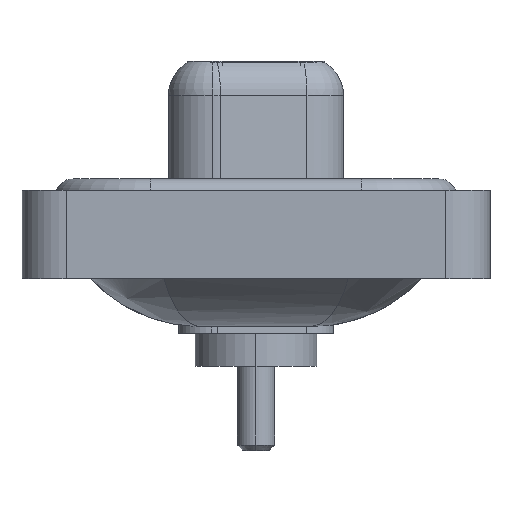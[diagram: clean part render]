
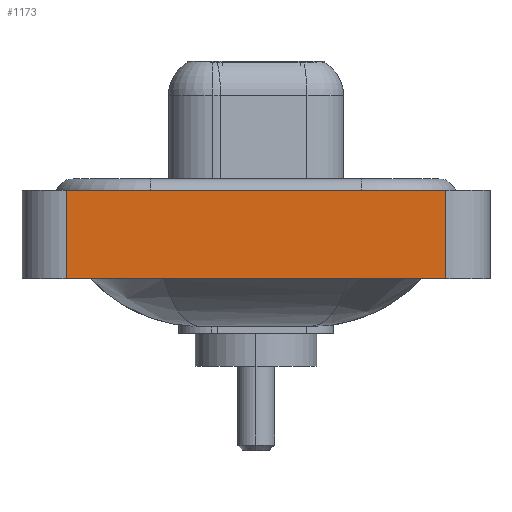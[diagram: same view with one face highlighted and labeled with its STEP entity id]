
A CAD part, left-side view. The second image highlights one B-rep face of the part: STEP entity #1173.
In plain terms, the highlighted planar face has unit normal (-1, 0, 0).
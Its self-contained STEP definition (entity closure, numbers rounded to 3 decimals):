
#1121 = LINE ( 'NONE', #6606, #13686 ) ;
#1173 = ADVANCED_FACE ( 'NONE', ( #10681 ), #9527, .T. ) ;
#1311 = LINE ( 'NONE', #13435, #8541 ) ;
#2403 = VERTEX_POINT ( 'NONE', #3202 ) ;
#3202 = CARTESIAN_POINT ( 'NONE',  ( -7.3, 8.55, 0.4 ) ) ;
#3320 = VERTEX_POINT ( 'NONE', #11436 ) ;
#3559 = DIRECTION ( 'NONE',  ( 0., 0., 1. ) ) ;
#3599 = EDGE_LOOP ( 'NONE', ( #17404, #8432, #3899, #7549 ) ) ;
#3883 = DIRECTION ( 'NONE',  ( 0., -1., 0. ) ) ;
#3899 = ORIENTED_EDGE ( 'NONE', *, *, #4424, .F. ) ;
#4030 = CARTESIAN_POINT ( 'NONE',  ( -7.3, -8.55, 0.4 ) ) ;
#4036 = VERTEX_POINT ( 'NONE', #15579 ) ;
#4424 = EDGE_CURVE ( 'NONE', #4036, #2403, #1311, .T. ) ;
#4844 = LINE ( 'NONE', #10255, #14801 ) ;
#6093 = EDGE_CURVE ( 'NONE', #3320, #15265, #13199, .T. ) ;
#6561 = EDGE_CURVE ( 'NONE', #2403, #15265, #1121, .T. ) ;
#6606 = CARTESIAN_POINT ( 'NONE',  ( -7.3, -8.55, 0.4 ) ) ;
#7549 = ORIENTED_EDGE ( 'NONE', *, *, #14933, .T. ) ;
#8340 = AXIS2_PLACEMENT_3D ( 'NONE', #15978, #10587, #14925 ) ;
#8432 = ORIENTED_EDGE ( 'NONE', *, *, #6561, .F. ) ;
#8541 = VECTOR ( 'NONE', #10956, 1000. ) ;
#9527 = PLANE ( 'NONE',  #8340 ) ;
#10255 = CARTESIAN_POINT ( 'NONE',  ( -7.3, -8.55, -3.6 ) ) ;
#10587 = DIRECTION ( 'NONE',  ( -1., 0., 0. ) ) ;
#10681 = FACE_OUTER_BOUND ( 'NONE', #3599, .T. ) ;
#10956 = DIRECTION ( 'NONE',  ( 0., 0., 1. ) ) ;
#11436 = CARTESIAN_POINT ( 'NONE',  ( -7.3, -8.55, -3.6 ) ) ;
#12024 = VECTOR ( 'NONE', #3559, 1000. ) ;
#13199 = LINE ( 'NONE', #17262, #12024 ) ;
#13435 = CARTESIAN_POINT ( 'NONE',  ( -7.3, 8.55, -3.6 ) ) ;
#13686 = VECTOR ( 'NONE', #17220, 1000. ) ;
#14801 = VECTOR ( 'NONE', #3883, 1000. ) ;
#14925 = DIRECTION ( 'NONE',  ( 0., 0., 1. ) ) ;
#14933 = EDGE_CURVE ( 'NONE', #4036, #3320, #4844, .T. ) ;
#15265 = VERTEX_POINT ( 'NONE', #4030 ) ;
#15579 = CARTESIAN_POINT ( 'NONE',  ( -7.3, 8.55, -3.6 ) ) ;
#15978 = CARTESIAN_POINT ( 'NONE',  ( -7.3, -8.55, -3.6 ) ) ;
#17220 = DIRECTION ( 'NONE',  ( 0., -1., 0. ) ) ;
#17262 = CARTESIAN_POINT ( 'NONE',  ( -7.3, -8.55, -3.6 ) ) ;
#17404 = ORIENTED_EDGE ( 'NONE', *, *, #6093, .T. ) ;
